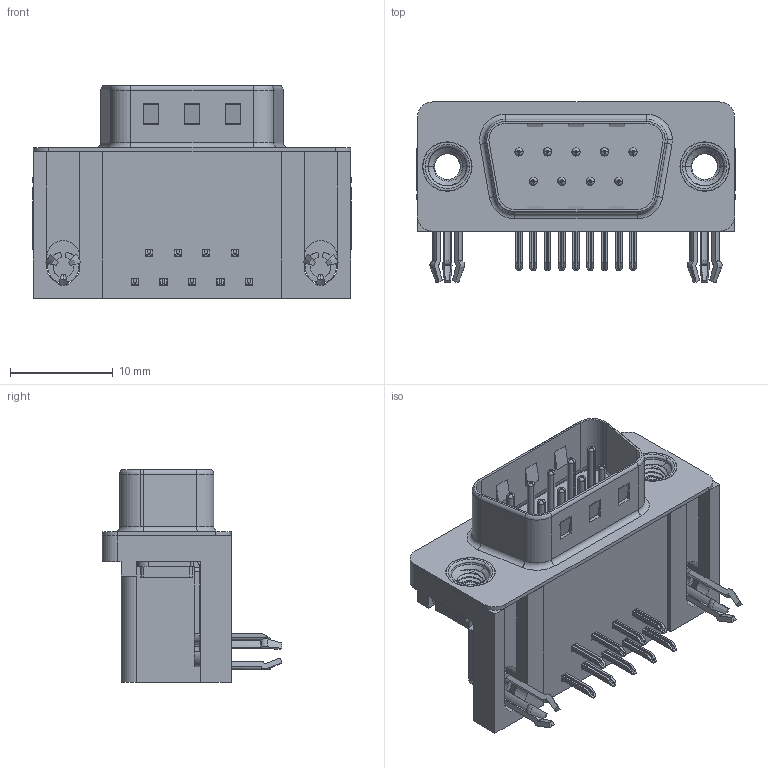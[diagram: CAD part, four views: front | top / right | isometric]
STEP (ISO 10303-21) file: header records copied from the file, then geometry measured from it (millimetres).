
FILE_DESCRIPTION (( 'STEP AP203' ), '1' );
FILE_NAME ('629-009-640-045.STEP', '2021-09-21T20:00:48', ( '' ), ( '' ), 'SwSTEP 2.0', 'SolidWorks 2020', '' );
FILE_SCHEMA (( 'CONFIG_CONTROL_DESIGN' ));
Length unit declared in the file: millimetre
Products named in the file (7): 629 M3 Threaded Rivet; 629 Housing_09 Socket; 629 3 Prong Board Lock; 629 Contact Top; 629-009-640-045; 629 Contact Bottom; 629 Shell_09 Socket
Assembly tree (15 placements, depth 2):
  629-009-640-045
    629 Housing_09 Socket
    629 Shell_09 Socket
    629 Contact Bottom  x4
    629 Contact Top  x5
    629 3 Prong Board Lock  x2
    629 M3 Threaded Rivet  x2
Bounding box: 30.89 x 17.48 x 20.6 mm (x, y, z)
Volume: 3724.8 mm3; surface area: 4822.3 mm2
Topology: 15 solids, 15 shells, 1093 faces, 2785 edges, 1747 vertices
Faces by surface type: plane 609, cylinder 325, torus 109, cone 44, bspline 6
Entity records: 17658 total; most frequent: CARTESIAN_POINT 4097, DIRECTION 2716, ORIENTED_EDGE 2592, EDGE_CURVE 1296, AXIS2_PLACEMENT_3D 948, VERTEX_POINT 828, LINE 820, VECTOR 820
